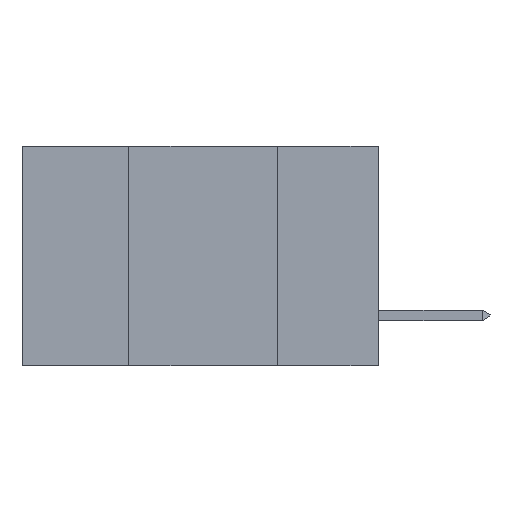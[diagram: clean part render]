
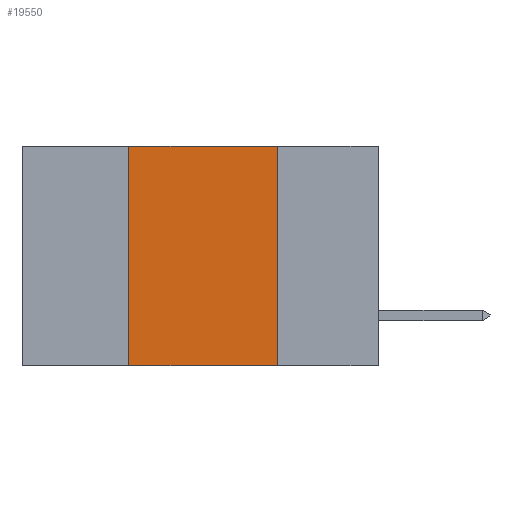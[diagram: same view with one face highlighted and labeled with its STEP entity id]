
A CAD part, left-side view. The second image highlights one B-rep face of the part: STEP entity #19550.
In plain terms, the highlighted planar face has unit normal (-1, 0, 0).
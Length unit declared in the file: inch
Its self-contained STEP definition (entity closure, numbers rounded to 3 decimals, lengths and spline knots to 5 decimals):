
#39 = CARTESIAN_POINT ( 'NONE',  ( 0., 0.6, 0. ) ) ;
#377 = VECTOR ( 'NONE', #3150, 39.37008 ) ;
#1529 = EDGE_CURVE ( 'NONE', #24378, #15233, #15967, .T. ) ;
#1755 = CARTESIAN_POINT ( 'NONE',  ( 0., 0.17, 0. ) ) ;
#2081 = DIRECTION ( 'NONE',  ( 0., 0., -1. ) ) ;
#2865 = EDGE_LOOP ( 'NONE', ( #11971, #18103, #7579, #24474 ) ) ;
#3150 = DIRECTION ( 'NONE',  ( 0., 0., -1. ) ) ;
#5134 = EDGE_CURVE ( 'NONE', #12615, #15233, #8401, .T. ) ;
#5720 = CARTESIAN_POINT ( 'NONE',  ( 0., 0.17, -0.37 ) ) ;
#6464 = CARTESIAN_POINT ( 'NONE',  ( 0., 0.42, 0. ) ) ;
#6747 = VECTOR ( 'NONE', #6754, 39.37008 ) ;
#6754 = DIRECTION ( 'NONE',  ( 0., -1., 0. ) ) ;
#7579 = ORIENTED_EDGE ( 'NONE', *, *, #20494, .F. ) ;
#7784 = PLANE ( 'NONE',  #9047 ) ;
#7942 = VERTEX_POINT ( 'NONE', #6464 ) ;
#8401 = LINE ( 'NONE', #14509, #377 ) ;
#9047 = AXIS2_PLACEMENT_3D ( 'NONE', #39, #21013, #2081 ) ;
#11200 = VECTOR ( 'NONE', #16007, 39.37008 ) ;
#11971 = ORIENTED_EDGE ( 'NONE', *, *, #5134, .F. ) ;
#12615 = VERTEX_POINT ( 'NONE', #1755 ) ;
#13330 = VECTOR ( 'NONE', #20840, 39.37008 ) ;
#13901 = CARTESIAN_POINT ( 'NONE',  ( 0., 0.6, 0. ) ) ;
#14509 = CARTESIAN_POINT ( 'NONE',  ( 0., 0.17, 0. ) ) ;
#15233 = VERTEX_POINT ( 'NONE', #5720 ) ;
#15967 = LINE ( 'NONE', #22885, #13330 ) ;
#16007 = DIRECTION ( 'NONE',  ( 0., 0., 1. ) ) ;
#18001 = LINE ( 'NONE', #19973, #11200 ) ;
#18103 = ORIENTED_EDGE ( 'NONE', *, *, #24190, .F. ) ;
#19550 = ADVANCED_FACE ( 'NONE', ( #20451 ), #7784, .F. ) ;
#19973 = CARTESIAN_POINT ( 'NONE',  ( 0., 0.42, 0. ) ) ;
#20451 = FACE_OUTER_BOUND ( 'NONE', #2865, .T. ) ;
#20494 = EDGE_CURVE ( 'NONE', #24378, #7942, #18001, .T. ) ;
#20840 = DIRECTION ( 'NONE',  ( 0., -1., 0. ) ) ;
#21013 = DIRECTION ( 'NONE',  ( 1., 0., 0. ) ) ;
#21609 = LINE ( 'NONE', #13901, #6747 ) ;
#22671 = CARTESIAN_POINT ( 'NONE',  ( 0., 0.42, -0.37 ) ) ;
#22885 = CARTESIAN_POINT ( 'NONE',  ( 0., 0.6, -0.37 ) ) ;
#24190 = EDGE_CURVE ( 'NONE', #7942, #12615, #21609, .T. ) ;
#24378 = VERTEX_POINT ( 'NONE', #22671 ) ;
#24474 = ORIENTED_EDGE ( 'NONE', *, *, #1529, .T. ) ;
